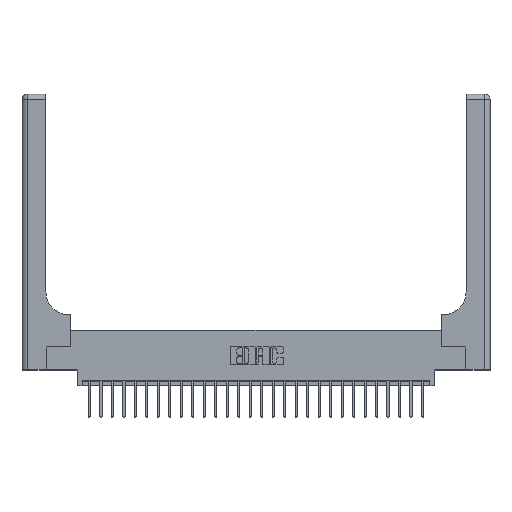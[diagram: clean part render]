
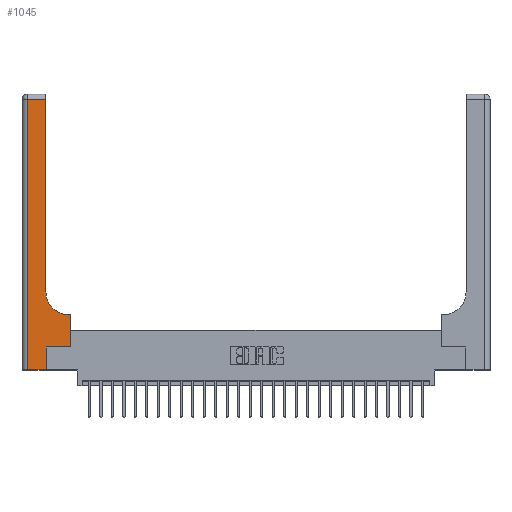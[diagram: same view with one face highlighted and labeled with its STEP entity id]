
A CAD part, top view. The second image highlights one B-rep face of the part: STEP entity #1045.
In plain terms, the highlighted planar face has unit normal (0, 0, 1).
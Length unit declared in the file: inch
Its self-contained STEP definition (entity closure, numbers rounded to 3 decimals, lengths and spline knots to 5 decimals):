
#455 = EDGE_CURVE ( 'NONE', #22366, #21104, #4582, .T. ) ;
#1045 = ADVANCED_FACE ( 'NONE', ( #6591 ), #10296, .F. ) ;
#1051 = LINE ( 'NONE', #13772, #19345 ) ;
#1347 = VERTEX_POINT ( 'NONE', #1760 ) ;
#1378 = VERTEX_POINT ( 'NONE', #23185 ) ;
#1431 = VERTEX_POINT ( 'NONE', #23589 ) ;
#1760 = CARTESIAN_POINT ( 'NONE',  ( 0.528, 0.25, 0.37 ) ) ;
#2104 = DIRECTION ( 'NONE',  ( 0., -1., 0. ) ) ;
#2293 = EDGE_CURVE ( 'NONE', #23838, #1378, #19047, .T. ) ;
#3060 = CARTESIAN_POINT ( 'NONE',  ( 0.528, 0.25, 0.37 ) ) ;
#3163 = VECTOR ( 'NONE', #3968, 39.37008 ) ;
#3473 = VERTEX_POINT ( 'NONE', #24620 ) ;
#3667 = ORIENTED_EDGE ( 'NONE', *, *, #12907, .T. ) ;
#3968 = DIRECTION ( 'NONE',  ( 0., 1., 0. ) ) ;
#4141 = CARTESIAN_POINT ( 'NONE',  ( 0., 3., 0.37 ) ) ;
#4269 = CARTESIAN_POINT ( 'NONE',  ( 0.51, 0.6, 0.37 ) ) ;
#4582 = CIRCLE ( 'NONE', #19859, 0.25 ) ;
#5509 = DIRECTION ( 'NONE',  ( -1., 0., 0. ) ) ;
#5517 = DIRECTION ( 'NONE',  ( 1., 0., 0. ) ) ;
#5913 = LINE ( 'NONE', #12225, #19494 ) ;
#6320 = DIRECTION ( 'NONE',  ( 0., 0., -1. ) ) ;
#6591 = FACE_OUTER_BOUND ( 'NONE', #22172, .T. ) ;
#7016 = ORIENTED_EDGE ( 'NONE', *, *, #12308, .T. ) ;
#7206 = EDGE_CURVE ( 'NONE', #25951, #3473, #16364, .T. ) ;
#7325 = VECTOR ( 'NONE', #2104, 39.37008 ) ;
#7360 = CARTESIAN_POINT ( 'NONE',  ( 0.528, 0.6, 0.37 ) ) ;
#8681 = DIRECTION ( 'NONE',  ( 0., 0., -1. ) ) ;
#8947 = CARTESIAN_POINT ( 'NONE',  ( 0.51, 0.85, 0.37 ) ) ;
#9116 = ORIENTED_EDGE ( 'NONE', *, *, #2293, .T. ) ;
#9806 = CARTESIAN_POINT ( 'NONE',  ( 0.26, 0.85, 0.37 ) ) ;
#10061 = VERTEX_POINT ( 'NONE', #7360 ) ;
#10296 = PLANE ( 'NONE',  #15992 ) ;
#10470 = CARTESIAN_POINT ( 'NONE',  ( 0.265, 0., 0.37 ) ) ;
#11012 = ORIENTED_EDGE ( 'NONE', *, *, #15662, .T. ) ;
#12225 = CARTESIAN_POINT ( 'NONE',  ( 0.265, 0.25, 0.37 ) ) ;
#12308 = EDGE_CURVE ( 'NONE', #10061, #22366, #16058, .T. ) ;
#12441 = EDGE_CURVE ( 'NONE', #1431, #23838, #20797, .T. ) ;
#12907 = EDGE_CURVE ( 'NONE', #21104, #1431, #16422, .T. ) ;
#13225 = DIRECTION ( 'NONE',  ( 1., 0., 0. ) ) ;
#13266 = CARTESIAN_POINT ( 'NONE',  ( 0.265, 0., 0.37 ) ) ;
#13307 = ORIENTED_EDGE ( 'NONE', *, *, #7206, .T. ) ;
#13772 = CARTESIAN_POINT ( 'NONE',  ( 0., 0., 0.37 ) ) ;
#14863 = DIRECTION ( 'NONE',  ( 0., 1., 0. ) ) ;
#15159 = VECTOR ( 'NONE', #26002, 39.37008 ) ;
#15662 = EDGE_CURVE ( 'NONE', #1378, #25951, #1051, .T. ) ;
#15949 = DIRECTION ( 'NONE',  ( 1., 0., 0. ) ) ;
#15992 = AXIS2_PLACEMENT_3D ( 'NONE', #4141, #6320, #18639 ) ;
#15994 = ORIENTED_EDGE ( 'NONE', *, *, #455, .T. ) ;
#16058 = LINE ( 'NONE', #26673, #23604 ) ;
#16364 = LINE ( 'NONE', #10470, #20080 ) ;
#16422 = LINE ( 'NONE', #24707, #3163 ) ;
#16865 = CARTESIAN_POINT ( 'NONE',  ( 0.06, 3., 0.37 ) ) ;
#17189 = ORIENTED_EDGE ( 'NONE', *, *, #20250, .T. ) ;
#18493 = DIRECTION ( 'NONE',  ( -1., 0., 0. ) ) ;
#18639 = DIRECTION ( 'NONE',  ( -1., 0., 0. ) ) ;
#18903 = CARTESIAN_POINT ( 'NONE',  ( 0., 2.94, 0.37 ) ) ;
#19047 = LINE ( 'NONE', #16865, #7325 ) ;
#19345 = VECTOR ( 'NONE', #15949, 39.37008 ) ;
#19494 = VECTOR ( 'NONE', #5517, 39.37008 ) ;
#19859 = AXIS2_PLACEMENT_3D ( 'NONE', #8947, #8681, #13225 ) ;
#20080 = VECTOR ( 'NONE', #14863, 39.37008 ) ;
#20250 = EDGE_CURVE ( 'NONE', #1347, #10061, #23802, .T. ) ;
#20797 = LINE ( 'NONE', #18903, #24049 ) ;
#21104 = VERTEX_POINT ( 'NONE', #9806 ) ;
#21485 = CARTESIAN_POINT ( 'NONE',  ( 0.06, 2.94, 0.37 ) ) ;
#22172 = EDGE_LOOP ( 'NONE', ( #3667, #26635, #9116, #11012, #13307, #26739, #17189, #7016, #15994 ) ) ;
#22366 = VERTEX_POINT ( 'NONE', #4269 ) ;
#23185 = CARTESIAN_POINT ( 'NONE',  ( 0.06, 0., 0.37 ) ) ;
#23499 = EDGE_CURVE ( 'NONE', #3473, #1347, #5913, .T. ) ;
#23589 = CARTESIAN_POINT ( 'NONE',  ( 0.26, 2.94, 0.37 ) ) ;
#23604 = VECTOR ( 'NONE', #5509, 39.37008 ) ;
#23802 = LINE ( 'NONE', #3060, #15159 ) ;
#23838 = VERTEX_POINT ( 'NONE', #21485 ) ;
#24049 = VECTOR ( 'NONE', #18493, 39.37008 ) ;
#24620 = CARTESIAN_POINT ( 'NONE',  ( 0.265, 0.25, 0.37 ) ) ;
#24707 = CARTESIAN_POINT ( 'NONE',  ( 0.26, 3., 0.37 ) ) ;
#25951 = VERTEX_POINT ( 'NONE', #13266 ) ;
#26002 = DIRECTION ( 'NONE',  ( 0., 1., 0. ) ) ;
#26635 = ORIENTED_EDGE ( 'NONE', *, *, #12441, .T. ) ;
#26673 = CARTESIAN_POINT ( 'NONE',  ( 0.26, 0.6, 0.37 ) ) ;
#26739 = ORIENTED_EDGE ( 'NONE', *, *, #23499, .T. ) ;
